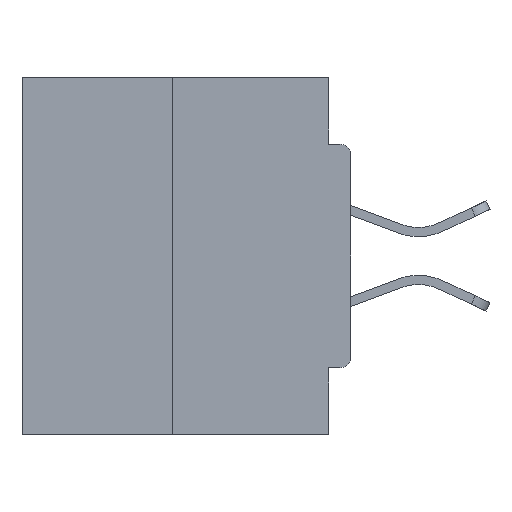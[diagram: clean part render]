
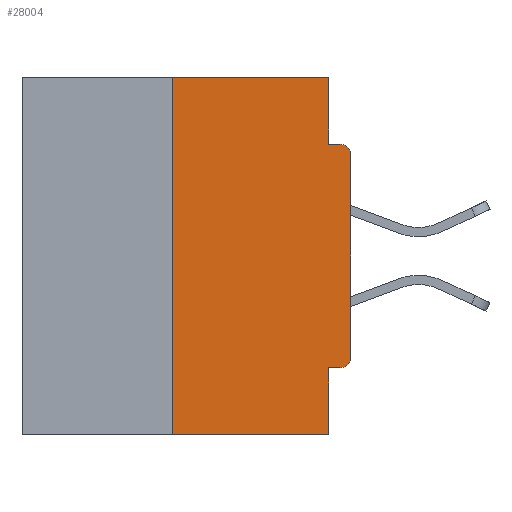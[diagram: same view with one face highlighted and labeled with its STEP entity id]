
A CAD part, left-side view. The second image highlights one B-rep face of the part: STEP entity #28004.
In plain terms, the highlighted planar face has unit normal (-1, 0, 0).
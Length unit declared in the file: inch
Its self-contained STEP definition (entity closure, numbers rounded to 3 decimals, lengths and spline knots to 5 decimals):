
#197 = CARTESIAN_POINT ( 'NONE',  ( 0., 0.25, 0. ) ) ;
#1968 = LINE ( 'NONE', #36883, #7083 ) ;
#4903 = CARTESIAN_POINT ( 'NONE',  ( 0., 0.46, -0.5 ) ) ;
#5149 = EDGE_CURVE ( 'NONE', #31507, #5276, #39943, .T. ) ;
#5276 = VERTEX_POINT ( 'NONE', #14727 ) ;
#7083 = VECTOR ( 'NONE', #26452, 39.37008 ) ;
#7497 = DIRECTION ( 'NONE',  ( 0., 0., -1. ) ) ;
#7972 = VERTEX_POINT ( 'NONE', #39147 ) ;
#8880 = ORIENTED_EDGE ( 'NONE', *, *, #12703, .F. ) ;
#9301 = ORIENTED_EDGE ( 'NONE', *, *, #35505, .T. ) ;
#10934 = DIRECTION ( 'NONE',  ( 0., 0., -1. ) ) ;
#11527 = VECTOR ( 'NONE', #20721, 39.37008 ) ;
#11785 = DIRECTION ( 'NONE',  ( 0., 0., -1. ) ) ;
#12231 = ORIENTED_EDGE ( 'NONE', *, *, #25191, .F. ) ;
#12547 = EDGE_CURVE ( 'NONE', #7972, #5276, #24268, .T. ) ;
#12703 = EDGE_CURVE ( 'NONE', #35259, #24138, #19151, .T. ) ;
#13251 = CARTESIAN_POINT ( 'NONE',  ( 0., 0.25, -0.5 ) ) ;
#13340 = EDGE_LOOP ( 'NONE', ( #8880, #12231, #17726, #36657, #24343, #9301, #20297, #33644, #32402, #35701 ) ) ;
#14116 = VERTEX_POINT ( 'NONE', #15915 ) ;
#14727 = CARTESIAN_POINT ( 'NONE',  ( 0., 0.015, -0.0935 ) ) ;
#15316 = LINE ( 'NONE', #35226, #38279 ) ;
#15825 = EDGE_CURVE ( 'NONE', #14116, #31507, #24028, .T. ) ;
#15915 = CARTESIAN_POINT ( 'NONE',  ( 0., 0., -0.3915 ) ) ;
#16678 = CARTESIAN_POINT ( 'NONE',  ( 0., 0.031, -0.5 ) ) ;
#16915 = CARTESIAN_POINT ( 'NONE',  ( 0., 0., 0. ) ) ;
#17468 = CARTESIAN_POINT ( 'NONE',  ( 0., 0.031, -0.5 ) ) ;
#17726 = ORIENTED_EDGE ( 'NONE', *, *, #39188, .T. ) ;
#18270 = DIRECTION ( 'NONE',  ( 0., -1., 0. ) ) ;
#18462 = CARTESIAN_POINT ( 'NONE',  ( 0., 0.46, 0. ) ) ;
#19151 = LINE ( 'NONE', #31623, #26294 ) ;
#20297 = ORIENTED_EDGE ( 'NONE', *, *, #15825, .T. ) ;
#20330 = CARTESIAN_POINT ( 'NONE',  ( 0., 0.015, -0.4065 ) ) ;
#20599 = DIRECTION ( 'NONE',  ( -1., 0., 0. ) ) ;
#20721 = DIRECTION ( 'NONE',  ( 0., -1., 0. ) ) ;
#22709 = VECTOR ( 'NONE', #23878, 39.37008 ) ;
#23173 = FACE_OUTER_BOUND ( 'NONE', #13340, .T. ) ;
#23310 = VERTEX_POINT ( 'NONE', #16678 ) ;
#23312 = DIRECTION ( 'NONE',  ( 0., 0., 1. ) ) ;
#23878 = DIRECTION ( 'NONE',  ( 0., -1., 0. ) ) ;
#23986 = DIRECTION ( 'NONE',  ( 0., 0., -1. ) ) ;
#24028 = LINE ( 'NONE', #16915, #36273 ) ;
#24138 = VERTEX_POINT ( 'NONE', #36965 ) ;
#24268 = LINE ( 'NONE', #37125, #11527 ) ;
#24343 = ORIENTED_EDGE ( 'NONE', *, *, #33725, .F. ) ;
#25089 = VECTOR ( 'NONE', #30445, 39.37008 ) ;
#25191 = EDGE_CURVE ( 'NONE', #41663, #35259, #15316, .T. ) ;
#25419 = AXIS2_PLACEMENT_3D ( 'NONE', #18462, #28258, #11785 ) ;
#26089 = EDGE_CURVE ( 'NONE', #24138, #7972, #1968, .T. ) ;
#26294 = VECTOR ( 'NONE', #18270, 39.37008 ) ;
#26452 = DIRECTION ( 'NONE',  ( 0., 0., -1. ) ) ;
#27016 = CARTESIAN_POINT ( 'NONE',  ( 0., 0.015, -0.3915 ) ) ;
#27410 = CARTESIAN_POINT ( 'NONE',  ( 0., 0.015, -0.1085 ) ) ;
#27541 = CARTESIAN_POINT ( 'NONE',  ( 0., 0.031, -0.4065 ) ) ;
#28004 = ADVANCED_FACE ( 'NONE', ( #23173 ), #38006, .F. ) ;
#28258 = DIRECTION ( 'NONE',  ( 1., 0., 0. ) ) ;
#28304 = VECTOR ( 'NONE', #10934, 39.37008 ) ;
#28563 = CARTESIAN_POINT ( 'NONE',  ( 0., 0., -0.1085 ) ) ;
#29310 = LINE ( 'NONE', #4903, #22709 ) ;
#30445 = DIRECTION ( 'NONE',  ( 0., 1., 0. ) ) ;
#30777 = AXIS2_PLACEMENT_3D ( 'NONE', #27016, #40397, #7497 ) ;
#31507 = VERTEX_POINT ( 'NONE', #28563 ) ;
#31623 = CARTESIAN_POINT ( 'NONE',  ( 0., 0.46, 0. ) ) ;
#31841 = EDGE_CURVE ( 'NONE', #37363, #23310, #41078, .T. ) ;
#32349 = DIRECTION ( 'NONE',  ( 0., 0., 1. ) ) ;
#32402 = ORIENTED_EDGE ( 'NONE', *, *, #12547, .F. ) ;
#32704 = VERTEX_POINT ( 'NONE', #20330 ) ;
#33324 = CARTESIAN_POINT ( 'NONE',  ( 0., 0., -0.4065 ) ) ;
#33644 = ORIENTED_EDGE ( 'NONE', *, *, #5149, .T. ) ;
#33725 = EDGE_CURVE ( 'NONE', #32704, #37363, #39383, .T. ) ;
#35226 = CARTESIAN_POINT ( 'NONE',  ( 0., 0.25, 0. ) ) ;
#35259 = VERTEX_POINT ( 'NONE', #197 ) ;
#35505 = EDGE_CURVE ( 'NONE', #32704, #14116, #37228, .T. ) ;
#35701 = ORIENTED_EDGE ( 'NONE', *, *, #26089, .F. ) ;
#36273 = VECTOR ( 'NONE', #23312, 39.37008 ) ;
#36657 = ORIENTED_EDGE ( 'NONE', *, *, #31841, .F. ) ;
#36883 = CARTESIAN_POINT ( 'NONE',  ( 0., 0.031, 0. ) ) ;
#36965 = CARTESIAN_POINT ( 'NONE',  ( 0., 0.031, 0. ) ) ;
#37125 = CARTESIAN_POINT ( 'NONE',  ( 0., 0., -0.0935 ) ) ;
#37228 = CIRCLE ( 'NONE', #30777, 0.015 ) ;
#37363 = VERTEX_POINT ( 'NONE', #27541 ) ;
#38006 = PLANE ( 'NONE',  #25419 ) ;
#38279 = VECTOR ( 'NONE', #32349, 39.37008 ) ;
#38521 = AXIS2_PLACEMENT_3D ( 'NONE', #27410, #20599, #23986 ) ;
#39147 = CARTESIAN_POINT ( 'NONE',  ( 0., 0.031, -0.0935 ) ) ;
#39188 = EDGE_CURVE ( 'NONE', #41663, #23310, #29310, .T. ) ;
#39383 = LINE ( 'NONE', #33324, #25089 ) ;
#39943 = CIRCLE ( 'NONE', #38521, 0.015 ) ;
#40397 = DIRECTION ( 'NONE',  ( -1., 0., 0. ) ) ;
#41078 = LINE ( 'NONE', #17468, #28304 ) ;
#41663 = VERTEX_POINT ( 'NONE', #13251 ) ;
